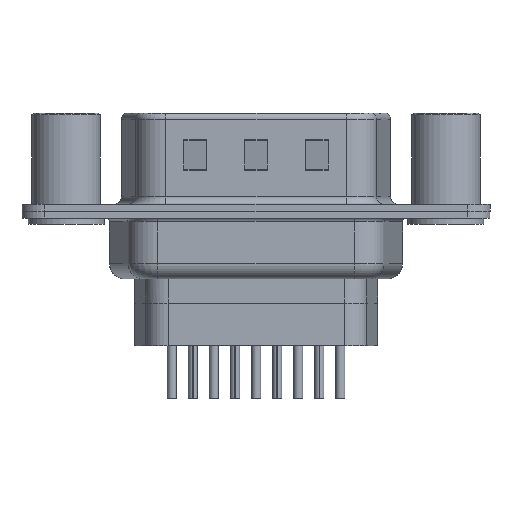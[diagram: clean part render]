
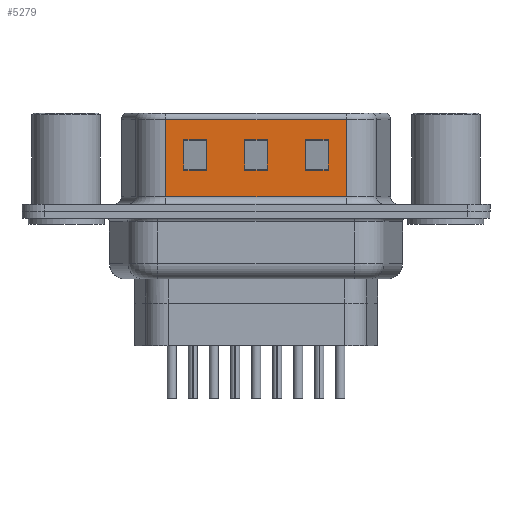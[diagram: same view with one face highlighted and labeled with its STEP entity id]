
A CAD part, front view. The second image highlights one B-rep face of the part: STEP entity #5279.
In plain terms, the highlighted planar face has unit normal (0, -1, 0).
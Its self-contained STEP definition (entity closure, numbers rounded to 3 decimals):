
#27 = CARTESIAN_POINT ( 'NONE',  ( 11.745, -4.58, 4.705 ) ) ;
#84 = DIRECTION ( 'NONE',  ( -1., 0., 0. ) ) ;
#246 = EDGE_CURVE ( 'NONE', #15882, #16978, #13463, .T. ) ;
#533 = VERTEX_POINT ( 'NONE', #10627 ) ;
#586 = VECTOR ( 'NONE', #4678, 1000. ) ;
#748 = DIRECTION ( 'NONE',  ( -1., 0., 0. ) ) ;
#814 = EDGE_CURVE ( 'NONE', #12127, #5334, #5577, .T. ) ;
#847 = VECTOR ( 'NONE', #16374, 1000. ) ;
#1183 = VERTEX_POINT ( 'NONE', #4731 ) ;
#1558 = DIRECTION ( 'NONE',  ( 1., 0., 0. ) ) ;
#1720 = VERTEX_POINT ( 'NONE', #14721 ) ;
#1982 = VERTEX_POINT ( 'NONE', #12931 ) ;
#2099 = LINE ( 'NONE', #14475, #9786 ) ;
#2259 = EDGE_CURVE ( 'NONE', #8203, #14462, #5606, .T. ) ;
#2400 = VECTOR ( 'NONE', #2669, 1000. ) ;
#2633 = DIRECTION ( 'NONE',  ( 0., 0., -1. ) ) ;
#2669 = DIRECTION ( 'NONE',  ( 0., 0., -1. ) ) ;
#2747 = DIRECTION ( 'NONE',  ( 0., 0., 1. ) ) ;
#2779 = EDGE_CURVE ( 'NONE', #12081, #1720, #16072, .T. ) ;
#3019 = ORIENTED_EDGE ( 'NONE', *, *, #6878, .T. ) ;
#3439 = DIRECTION ( 'NONE',  ( 0., 0., -1. ) ) ;
#4267 = VECTOR ( 'NONE', #1558, 1000. ) ;
#4574 = CARTESIAN_POINT ( 'NONE',  ( 17.245, -4.58, 6.52 ) ) ;
#4678 = DIRECTION ( 'NONE',  ( 0., 0., -1. ) ) ;
#4731 = CARTESIAN_POINT ( 'NONE',  ( 7.745, -4.58, 2.705 ) ) ;
#4757 = ORIENTED_EDGE ( 'NONE', *, *, #16331, .T. ) ;
#4975 = LINE ( 'NONE', #11266, #12386 ) ;
#5061 = ORIENTED_EDGE ( 'NONE', *, *, #16575, .T. ) ;
#5279 = ADVANCED_FACE ( 'NONE', ( #14900, #18383, #7054, #7466 ), #13357, .F. ) ;
#5334 = VERTEX_POINT ( 'NONE', #9116 ) ;
#5405 = CARTESIAN_POINT ( 'NONE',  ( 13.245, -4.58, 4.705 ) ) ;
#5449 = VECTOR ( 'NONE', #11046, 1000. ) ;
#5531 = CARTESIAN_POINT ( 'NONE',  ( 18.445, -4.58, 6.02 ) ) ;
#5577 = LINE ( 'NONE', #11947, #6369 ) ;
#5582 = CARTESIAN_POINT ( 'NONE',  ( 9.245, -4.58, 4.705 ) ) ;
#5606 = LINE ( 'NONE', #18541, #4267 ) ;
#5616 = DIRECTION ( 'NONE',  ( 0., 0., 1. ) ) ;
#5706 = EDGE_CURVE ( 'NONE', #15705, #15377, #14037, .T. ) ;
#5790 = VERTEX_POINT ( 'NONE', #27 ) ;
#5910 = EDGE_LOOP ( 'NONE', ( #7124, #19374, #4757, #19797 ) ) ;
#6369 = VECTOR ( 'NONE', #16502, 1000. ) ;
#6635 = DIRECTION ( 'NONE',  ( 1., 0., 0. ) ) ;
#6729 = EDGE_CURVE ( 'NONE', #15200, #12127, #10867, .T. ) ;
#6878 = EDGE_CURVE ( 'NONE', #5790, #15304, #2099, .T. ) ;
#7017 = EDGE_LOOP ( 'NONE', ( #3019, #5061, #17189, #9858 ) ) ;
#7054 = FACE_BOUND ( 'NONE', #7017, .T. ) ;
#7116 = VECTOR ( 'NONE', #14060, 1000. ) ;
#7124 = ORIENTED_EDGE ( 'NONE', *, *, #10392, .T. ) ;
#7282 = CARTESIAN_POINT ( 'NONE',  ( 15.745, -4.58, 4.705 ) ) ;
#7346 = CARTESIAN_POINT ( 'NONE',  ( 15.745, -4.58, 2.705 ) ) ;
#7451 = VECTOR ( 'NONE', #2747, 1000. ) ;
#7466 = FACE_OUTER_BOUND ( 'NONE', #9878, .T. ) ;
#7475 = LINE ( 'NONE', #5531, #8409 ) ;
#7625 = ORIENTED_EDGE ( 'NONE', *, *, #16881, .T. ) ;
#7638 = CARTESIAN_POINT ( 'NONE',  ( 22.445, -4.58, 2.705 ) ) ;
#7838 = CARTESIAN_POINT ( 'NONE',  ( 6.545, -4.58, 0.95 ) ) ;
#7845 = ORIENTED_EDGE ( 'NONE', *, *, #814, .T. ) ;
#8107 = VECTOR ( 'NONE', #2633, 1000. ) ;
#8203 = VERTEX_POINT ( 'NONE', #18877 ) ;
#8409 = VECTOR ( 'NONE', #12205, 1000. ) ;
#9116 = CARTESIAN_POINT ( 'NONE',  ( 18.445, -4.58, 0.95 ) ) ;
#9173 = VECTOR ( 'NONE', #748, 1000. ) ;
#9393 = EDGE_CURVE ( 'NONE', #533, #1183, #11657, .T. ) ;
#9452 = ORIENTED_EDGE ( 'NONE', *, *, #13058, .T. ) ;
#9786 = VECTOR ( 'NONE', #6635, 1000. ) ;
#9858 = ORIENTED_EDGE ( 'NONE', *, *, #11640, .T. ) ;
#9878 = EDGE_LOOP ( 'NONE', ( #13436, #12610, #10095, #7845 ) ) ;
#10095 = ORIENTED_EDGE ( 'NONE', *, *, #6729, .T. ) ;
#10352 = DIRECTION ( 'NONE',  ( 0., 0., 1. ) ) ;
#10392 = EDGE_CURVE ( 'NONE', #16978, #15705, #13641, .T. ) ;
#10456 = CARTESIAN_POINT ( 'NONE',  ( 18.445, -4.58, 6.52 ) ) ;
#10491 = CARTESIAN_POINT ( 'NONE',  ( 9.245, -4.58, 6.52 ) ) ;
#10627 = CARTESIAN_POINT ( 'NONE',  ( 9.245, -4.58, 2.705 ) ) ;
#10867 = LINE ( 'NONE', #18802, #586 ) ;
#11046 = DIRECTION ( 'NONE',  ( -1., 0., 0. ) ) ;
#11266 = CARTESIAN_POINT ( 'NONE',  ( 13.245, -4.58, 6.52 ) ) ;
#11614 = CARTESIAN_POINT ( 'NONE',  ( 11.745, -4.58, 6.52 ) ) ;
#11640 = EDGE_CURVE ( 'NONE', #1720, #5790, #19669, .T. ) ;
#11657 = LINE ( 'NONE', #19601, #9173 ) ;
#11696 = LINE ( 'NONE', #17984, #18640 ) ;
#11947 = CARTESIAN_POINT ( 'NONE',  ( 18.445, -4.58, 0.95 ) ) ;
#12081 = VERTEX_POINT ( 'NONE', #16823 ) ;
#12104 = DIRECTION ( 'NONE',  ( 1., 0., 0. ) ) ;
#12121 = LINE ( 'NONE', #18011, #7451 ) ;
#12127 = VERTEX_POINT ( 'NONE', #7838 ) ;
#12205 = DIRECTION ( 'NONE',  ( -1., 0., 0. ) ) ;
#12386 = VECTOR ( 'NONE', #3439, 1000. ) ;
#12610 = ORIENTED_EDGE ( 'NONE', *, *, #20360, .T. ) ;
#12899 = ORIENTED_EDGE ( 'NONE', *, *, #2259, .T. ) ;
#12931 = CARTESIAN_POINT ( 'NONE',  ( 18.445, -4.58, 6.02 ) ) ;
#13058 = EDGE_CURVE ( 'NONE', #14462, #533, #18024, .T. ) ;
#13307 = ORIENTED_EDGE ( 'NONE', *, *, #9393, .T. ) ;
#13357 = PLANE ( 'NONE',  #19672 ) ;
#13436 = ORIENTED_EDGE ( 'NONE', *, *, #18256, .F. ) ;
#13463 = LINE ( 'NONE', #17996, #14915 ) ;
#13641 = LINE ( 'NONE', #4574, #7116 ) ;
#13974 = CARTESIAN_POINT ( 'NONE',  ( 17.245, -4.58, 4.705 ) ) ;
#14037 = LINE ( 'NONE', #7638, #5449 ) ;
#14060 = DIRECTION ( 'NONE',  ( 0., 0., -1. ) ) ;
#14462 = VERTEX_POINT ( 'NONE', #5582 ) ;
#14475 = CARTESIAN_POINT ( 'NONE',  ( 18.445, -4.58, 4.705 ) ) ;
#14721 = CARTESIAN_POINT ( 'NONE',  ( 11.745, -4.58, 2.705 ) ) ;
#14900 = FACE_BOUND ( 'NONE', #15798, .T. ) ;
#14915 = VECTOR ( 'NONE', #12104, 1000. ) ;
#15200 = VERTEX_POINT ( 'NONE', #19028 ) ;
#15304 = VERTEX_POINT ( 'NONE', #5405 ) ;
#15362 = VECTOR ( 'NONE', #84, 1000. ) ;
#15377 = VERTEX_POINT ( 'NONE', #7346 ) ;
#15705 = VERTEX_POINT ( 'NONE', #17450 ) ;
#15798 = EDGE_LOOP ( 'NONE', ( #9452, #13307, #7625, #12899 ) ) ;
#15882 = VERTEX_POINT ( 'NONE', #7282 ) ;
#16072 = LINE ( 'NONE', #17491, #15362 ) ;
#16331 = EDGE_CURVE ( 'NONE', #15377, #15882, #11696, .T. ) ;
#16374 = DIRECTION ( 'NONE',  ( 0., 0., 1. ) ) ;
#16502 = DIRECTION ( 'NONE',  ( 1., 0., 0. ) ) ;
#16575 = EDGE_CURVE ( 'NONE', #15304, #12081, #4975, .T. ) ;
#16823 = CARTESIAN_POINT ( 'NONE',  ( 13.245, -4.58, 2.705 ) ) ;
#16881 = EDGE_CURVE ( 'NONE', #1183, #8203, #12121, .T. ) ;
#16978 = VERTEX_POINT ( 'NONE', #13974 ) ;
#17189 = ORIENTED_EDGE ( 'NONE', *, *, #2779, .T. ) ;
#17450 = CARTESIAN_POINT ( 'NONE',  ( 17.245, -4.58, 2.705 ) ) ;
#17491 = CARTESIAN_POINT ( 'NONE',  ( 18.445, -4.58, 2.705 ) ) ;
#17984 = CARTESIAN_POINT ( 'NONE',  ( 15.745, -4.58, 6.52 ) ) ;
#17996 = CARTESIAN_POINT ( 'NONE',  ( 22.445, -4.58, 4.705 ) ) ;
#18011 = CARTESIAN_POINT ( 'NONE',  ( 7.745, -4.58, 6.52 ) ) ;
#18024 = LINE ( 'NONE', #10491, #2400 ) ;
#18256 = EDGE_CURVE ( 'NONE', #1982, #5334, #19743, .T. ) ;
#18383 = FACE_BOUND ( 'NONE', #5910, .T. ) ;
#18541 = CARTESIAN_POINT ( 'NONE',  ( 14.445, -4.58, 4.705 ) ) ;
#18640 = VECTOR ( 'NONE', #5616, 1000. ) ;
#18802 = CARTESIAN_POINT ( 'NONE',  ( 6.545, -4.58, 6.52 ) ) ;
#18877 = CARTESIAN_POINT ( 'NONE',  ( 7.745, -4.58, 4.705 ) ) ;
#19028 = CARTESIAN_POINT ( 'NONE',  ( 6.545, -4.58, 6.02 ) ) ;
#19374 = ORIENTED_EDGE ( 'NONE', *, *, #5706, .T. ) ;
#19601 = CARTESIAN_POINT ( 'NONE',  ( 14.445, -4.58, 2.705 ) ) ;
#19669 = LINE ( 'NONE', #11614, #847 ) ;
#19672 = AXIS2_PLACEMENT_3D ( 'NONE', #19934, #19829, #10352 ) ;
#19743 = LINE ( 'NONE', #10456, #8107 ) ;
#19797 = ORIENTED_EDGE ( 'NONE', *, *, #246, .T. ) ;
#19829 = DIRECTION ( 'NONE',  ( 0., 1., 0. ) ) ;
#19934 = CARTESIAN_POINT ( 'NONE',  ( 18.445, -4.58, 6.52 ) ) ;
#20360 = EDGE_CURVE ( 'NONE', #1982, #15200, #7475, .T. ) ;
